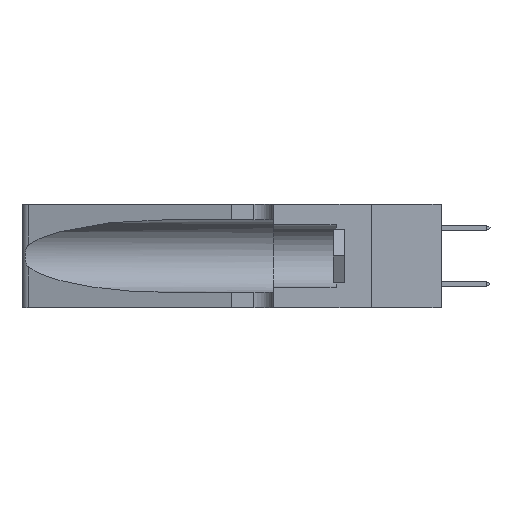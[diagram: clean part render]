
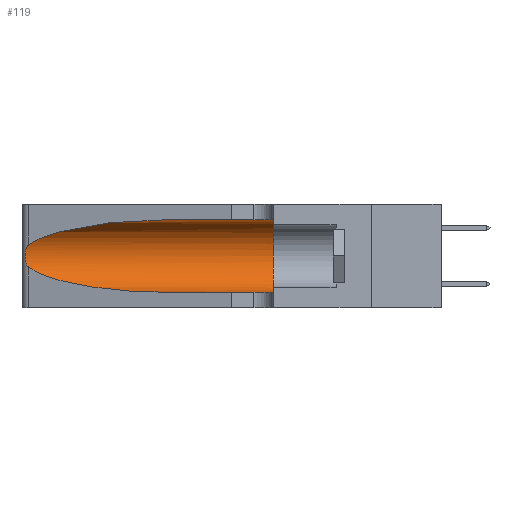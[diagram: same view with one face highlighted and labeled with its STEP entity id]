
A CAD part, left-side view. The second image highlights one B-rep face of the part: STEP entity #119.
In plain terms, the highlighted cylindrical face has radius 3.308 mm (diameter 6.617 mm), a partial arc.
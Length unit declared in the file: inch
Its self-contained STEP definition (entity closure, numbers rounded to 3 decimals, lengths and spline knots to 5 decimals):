
#69 = DIRECTION ( 'NONE',  ( 0., 0., -1. ) ) ;
#119 = ADVANCED_FACE ( 'NONE', ( #18537 ), #17567, .F. ) ;
#299 = VERTEX_POINT ( 'NONE', #515 ) ;
#424 = CARTESIAN_POINT ( 'NONE',  ( 0.26075, 1.23896, 0.178 ) ) ;
#515 = CARTESIAN_POINT ( 'NONE',  ( 0.25487, 1.22718, 0.22369 ) ) ;
#647 = CIRCLE ( 'NONE', #19558, 0.13025 ) ;
#915 = B_SPLINE_CURVE_WITH_KNOTS ( 'NONE', 3,
 ( #5206, #13006, #6784, #17667, #8362, #19221, #9925, #424, #11508, #2068, #13076, #3666, #14645, #5273 ),
 .UNSPECIFIED., .F., .F.,
 ( 4, 2, 2, 2, 2, 2, 4 ),
 ( 0., 0.00027, 0.00053, 0.00107, 0.0016, 0.00187, 0.00214 ),
 .UNSPECIFIED. ) ;
#1209 = VERTEX_POINT ( 'NONE', #12114 ) ;
#1713 =( BOUNDED_CURVE ( )  B_SPLINE_CURVE ( 3, ( #8070, #3291, #11211, #1760 ),
 .UNSPECIFIED., .F., .F. ) 
 B_SPLINE_CURVE_WITH_KNOTS ( ( 4, 4 ),
 ( 1.5708, 2.84003 ),
 .UNSPECIFIED. ) 
 CURVE ( )  GEOMETRIC_REPRESENTATION_ITEM ( )  RATIONAL_B_SPLINE_CURVE ( ( 1., 0.87, 0.87, 1. ) ) 
 REPRESENTATION_ITEM ( '' )  );
#1760 = CARTESIAN_POINT ( 'NONE',  ( 0.25487, 1.22718, 0.22369 ) ) ;
#2068 = CARTESIAN_POINT ( 'NONE',  ( 0.25856, 1.23593, 0.16098 ) ) ;
#2471 = CARTESIAN_POINT ( 'NONE',  ( 0.25487, 1.22718, 0.14631 ) ) ;
#2539 = EDGE_LOOP ( 'NONE', ( #9854, #8888, #4667, #11328, #4727, #19776 ) ) ;
#2740 =( BOUNDED_CURVE ( )  B_SPLINE_CURVE ( 3, ( #2471, #11886, #15014, #5673 ),
 .UNSPECIFIED., .F., .T. ) 
 B_SPLINE_CURVE_WITH_KNOTS ( ( 4, 4 ),
 ( 3.44316, 4.71239 ),
 .UNSPECIFIED. ) 
 CURVE ( )  GEOMETRIC_REPRESENTATION_ITEM ( )  RATIONAL_B_SPLINE_CURVE ( ( 1., 0.87, 0.87, 1. ) ) 
 REPRESENTATION_ITEM ( '' )  );
#3086 = VERTEX_POINT ( 'NONE', #13615 ) ;
#3132 = LINE ( 'NONE', #9889, #19264 ) ;
#3225 = CARTESIAN_POINT ( 'NONE',  ( 0.1305, 0.35, 0.31525 ) ) ;
#3271 = CARTESIAN_POINT ( 'NONE',  ( 0.1305, 0.35, 0.185 ) ) ;
#3291 = CARTESIAN_POINT ( 'NONE',  ( 0.18966, 0.96281, 0.31525 ) ) ;
#3666 = CARTESIAN_POINT ( 'NONE',  ( 0.25639, 1.23186, 0.15144 ) ) ;
#4588 = EDGE_CURVE ( 'NONE', #3086, #5592, #2740, .T. ) ;
#4626 = DIRECTION ( 'NONE',  ( 0., -1., 0. ) ) ;
#4667 = ORIENTED_EDGE ( 'NONE', *, *, #4588, .T. ) ;
#4727 = ORIENTED_EDGE ( 'NONE', *, *, #7348, .F. ) ;
#4796 = CARTESIAN_POINT ( 'NONE',  ( 0.1305, 0.35, 0.05475 ) ) ;
#4885 = DIRECTION ( 'NONE',  ( 0., 0., 1. ) ) ;
#5206 = CARTESIAN_POINT ( 'NONE',  ( 0.25487, 1.22718, 0.22369 ) ) ;
#5227 = DIRECTION ( 'NONE',  ( 0., -1., 0. ) ) ;
#5273 = CARTESIAN_POINT ( 'NONE',  ( 0.25487, 1.22718, 0.14631 ) ) ;
#5592 = VERTEX_POINT ( 'NONE', #7823 ) ;
#5673 = CARTESIAN_POINT ( 'NONE',  ( 0.1305, 0.72297, 0.05475 ) ) ;
#6784 = CARTESIAN_POINT ( 'NONE',  ( 0.25639, 1.23184, 0.21858 ) ) ;
#7348 = EDGE_CURVE ( 'NONE', #16833, #13022, #647, .T. ) ;
#7823 = CARTESIAN_POINT ( 'NONE',  ( 0.1305, 0.72297, 0.05475 ) ) ;
#8070 = CARTESIAN_POINT ( 'NONE',  ( 0.1305, 0.72297, 0.31525 ) ) ;
#8362 = CARTESIAN_POINT ( 'NONE',  ( 0.25854, 1.2359, 0.20912 ) ) ;
#8888 = ORIENTED_EDGE ( 'NONE', *, *, #18146, .T. ) ;
#9854 = ORIENTED_EDGE ( 'NONE', *, *, #16864, .T. ) ;
#9889 = CARTESIAN_POINT ( 'NONE',  ( 0.1305, 1.61858, 0.31525 ) ) ;
#9925 = CARTESIAN_POINT ( 'NONE',  ( 0.26075, 1.23896, 0.19203 ) ) ;
#11044 = AXIS2_PLACEMENT_3D ( 'NONE', #12828, #4626, #69 ) ;
#11211 = CARTESIAN_POINT ( 'NONE',  ( 0.2373, 1.15595, 0.28018 ) ) ;
#11274 = DIRECTION ( 'NONE',  ( 0., -1., 0. ) ) ;
#11328 = ORIENTED_EDGE ( 'NONE', *, *, #18935, .T. ) ;
#11508 = CARTESIAN_POINT ( 'NONE',  ( 0.26017, 1.23833, 0.17102 ) ) ;
#11886 = CARTESIAN_POINT ( 'NONE',  ( 0.2373, 1.15595, 0.08982 ) ) ;
#12114 = CARTESIAN_POINT ( 'NONE',  ( 0.1305, 0.72297, 0.31525 ) ) ;
#12828 = CARTESIAN_POINT ( 'NONE',  ( 0.1305, 1.61858, 0.185 ) ) ;
#13006 = CARTESIAN_POINT ( 'NONE',  ( 0.25555, 1.22994, 0.2215 ) ) ;
#13022 = VERTEX_POINT ( 'NONE', #4796 ) ;
#13076 = CARTESIAN_POINT ( 'NONE',  ( 0.25789, 1.23486, 0.15765 ) ) ;
#13615 = CARTESIAN_POINT ( 'NONE',  ( 0.25487, 1.22718, 0.14631 ) ) ;
#14239 = DIRECTION ( 'NONE',  ( 0., 1., 0. ) ) ;
#14428 = EDGE_CURVE ( 'NONE', #1209, #16833, #3132, .T. ) ;
#14645 = CARTESIAN_POINT ( 'NONE',  ( 0.25555, 1.22993, 0.14849 ) ) ;
#15014 = CARTESIAN_POINT ( 'NONE',  ( 0.18966, 0.96281, 0.05475 ) ) ;
#15839 = VECTOR ( 'NONE', #11274, 39.37008 ) ;
#16833 = VERTEX_POINT ( 'NONE', #3225 ) ;
#16864 = EDGE_CURVE ( 'NONE', #1209, #299, #1713, .T. ) ;
#17567 = CYLINDRICAL_SURFACE ( 'NONE', #11044, 0.13025 ) ;
#17667 = CARTESIAN_POINT ( 'NONE',  ( 0.25787, 1.23484, 0.2124 ) ) ;
#18146 = EDGE_CURVE ( 'NONE', #299, #3086, #915, .T. ) ;
#18537 = FACE_OUTER_BOUND ( 'NONE', #2539, .T. ) ;
#18925 = CARTESIAN_POINT ( 'NONE',  ( 0.1305, 1.61858, 0.05475 ) ) ;
#18935 = EDGE_CURVE ( 'NONE', #5592, #13022, #19936, .T. ) ;
#19221 = CARTESIAN_POINT ( 'NONE',  ( 0.26018, 1.23835, 0.19895 ) ) ;
#19264 = VECTOR ( 'NONE', #5227, 39.37008 ) ;
#19558 = AXIS2_PLACEMENT_3D ( 'NONE', #3271, #14239, #4885 ) ;
#19776 = ORIENTED_EDGE ( 'NONE', *, *, #14428, .F. ) ;
#19936 = LINE ( 'NONE', #18925, #15839 ) ;
